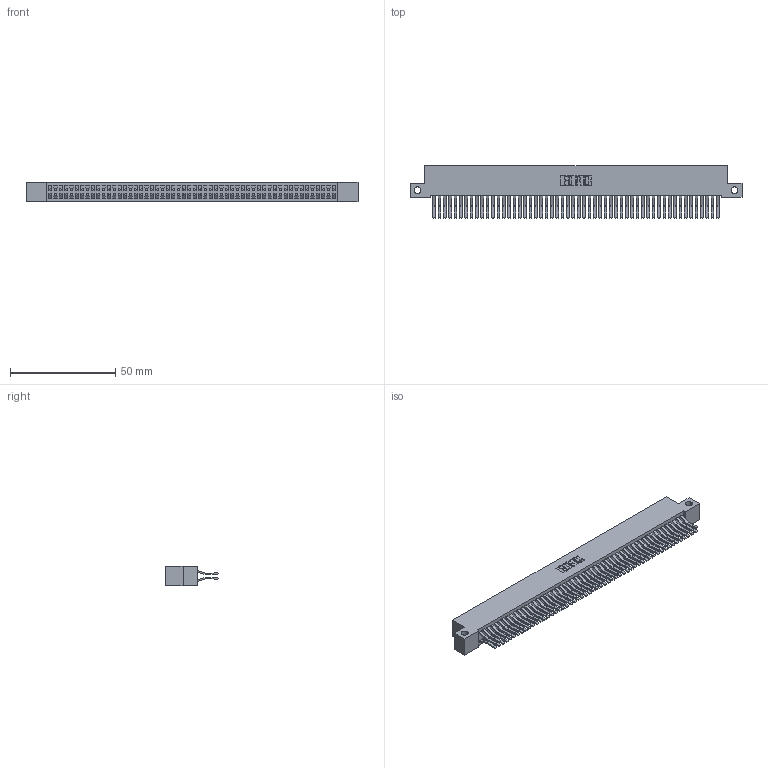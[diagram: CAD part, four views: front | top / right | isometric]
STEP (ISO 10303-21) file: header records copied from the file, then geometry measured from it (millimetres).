
FILE_DESCRIPTION (( 'STEP AP203' ), '1' );
FILE_NAME ('392-108-560-212.STEP', '2019-10-09T23:31:12', ( '' ), ( '' ), 'SwSTEP 2.0', 'SolidWorks 2016', '' );
FILE_SCHEMA (( 'CONFIG_CONTROL_DESIGN' ));
Length unit declared in the file: inch
Products named in the file (3): 342 Part_Side Mount; 345-292-001_560 Tail; 392-108-560-212
Assembly tree (109 placements, depth 2):
  392-108-560-212
    342 Part_Side Mount
    345-292-001_560 Tail  x108
Bounding box: 157.48 x 24.78 x 9.4 mm (x, y, z)
Volume: 14841.5 mm3; surface area: 25994.4 mm2
Topology: 109 solids, 109 shells, 5942 faces, 17687 edges, 11646 vertices
Faces by surface type: plane 3954, cylinder 1988
Entity records: 33147 total; most frequent: CARTESIAN_POINT 5478, ORIENTED_EDGE 5414, DIRECTION 4663, EDGE_CURVE 2707, LINE 2575, VECTOR 2575, VERTEX_POINT 1802, AXIS2_PLACEMENT_3D 1044
